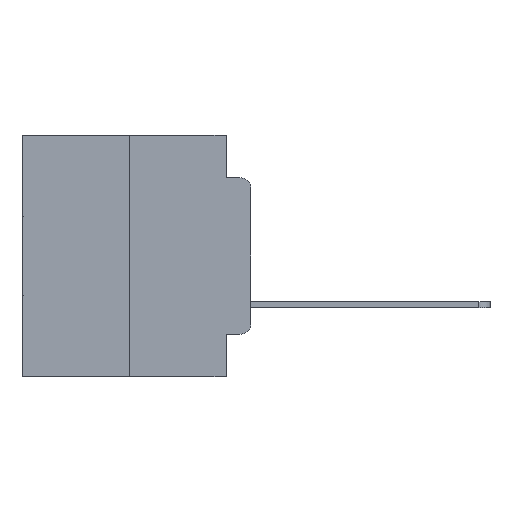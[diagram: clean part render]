
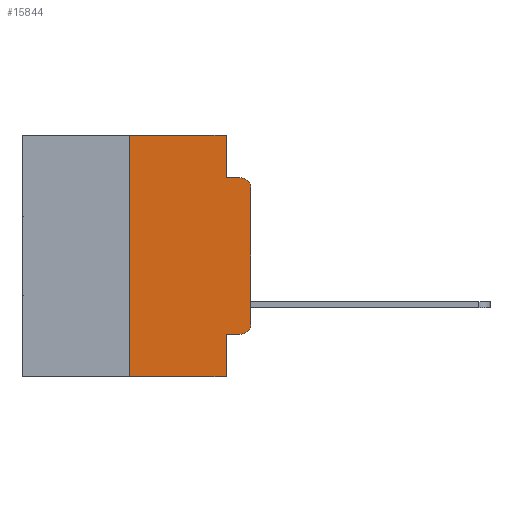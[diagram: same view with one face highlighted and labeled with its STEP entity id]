
A CAD part, left-side view. The second image highlights one B-rep face of the part: STEP entity #15844.
In plain terms, the highlighted planar face has unit normal (-1, 0, 0).
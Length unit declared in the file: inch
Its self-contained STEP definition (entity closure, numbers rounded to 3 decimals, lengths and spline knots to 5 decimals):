
#1087 = LINE ( 'NONE', #21592, #25274 ) ;
#2406 = AXIS2_PLACEMENT_3D ( 'NONE', #21463, #7665, #23724 ) ;
#2684 = CIRCLE ( 'NONE', #2406, 0.02 ) ;
#3044 = VECTOR ( 'NONE', #12171, 39.37008 ) ;
#3562 = EDGE_CURVE ( 'NONE', #9791, #24320, #6657, .T. ) ;
#3823 = LINE ( 'NONE', #4942, #3044 ) ;
#4385 = LINE ( 'NONE', #28917, #22219 ) ;
#4664 = CARTESIAN_POINT ( 'NONE',  ( 0., 0.051, 0. ) ) ;
#4942 = CARTESIAN_POINT ( 'NONE',  ( 0., 0.051, 0. ) ) ;
#5201 = DIRECTION ( 'NONE',  ( 0., 0., 1. ) ) ;
#5294 = EDGE_CURVE ( 'NONE', #24320, #14444, #12164, .T. ) ;
#6011 = EDGE_CURVE ( 'NONE', #27297, #16325, #13536, .T. ) ;
#6657 = CIRCLE ( 'NONE', #10305, 0.02 ) ;
#6861 = VERTEX_POINT ( 'NONE', #24099 ) ;
#6896 = FACE_OUTER_BOUND ( 'NONE', #25706, .T. ) ;
#7262 = VECTOR ( 'NONE', #14156, 39.37008 ) ;
#7665 = DIRECTION ( 'NONE',  ( -1., 0., 0. ) ) ;
#7783 = LINE ( 'NONE', #19919, #13334 ) ;
#7862 = LINE ( 'NONE', #29389, #29689 ) ;
#9021 = ORIENTED_EDGE ( 'NONE', *, *, #5294, .T. ) ;
#9426 = CARTESIAN_POINT ( 'NONE',  ( 0., 0.051, -0.4115 ) ) ;
#9547 = CARTESIAN_POINT ( 'NONE',  ( 0., 0.02, -0.0885 ) ) ;
#9785 = DIRECTION ( 'NONE',  ( 0., 0., -1. ) ) ;
#9791 = VERTEX_POINT ( 'NONE', #19637 ) ;
#9823 = CARTESIAN_POINT ( 'NONE',  ( 0., 0.25, -0.5 ) ) ;
#9932 = CARTESIAN_POINT ( 'NONE',  ( 0., 0., -0.3915 ) ) ;
#10040 = ORIENTED_EDGE ( 'NONE', *, *, #14467, .T. ) ;
#10305 = AXIS2_PLACEMENT_3D ( 'NONE', #21057, #21060, #21267 ) ;
#10607 = PLANE ( 'NONE',  #10878 ) ;
#10878 = AXIS2_PLACEMENT_3D ( 'NONE', #26348, #28483, #15251 ) ;
#11015 = ORIENTED_EDGE ( 'NONE', *, *, #29801, .F. ) ;
#11529 = EDGE_CURVE ( 'NONE', #25397, #9791, #4385, .T. ) ;
#11593 = DIRECTION ( 'NONE',  ( 0., -1., 0. ) ) ;
#12084 = ORIENTED_EDGE ( 'NONE', *, *, #15018, .F. ) ;
#12164 = LINE ( 'NONE', #27948, #16884 ) ;
#12171 = DIRECTION ( 'NONE',  ( 0., 0., -1. ) ) ;
#12251 = CARTESIAN_POINT ( 'NONE',  ( 0., 0., -0.1085 ) ) ;
#12351 = ORIENTED_EDGE ( 'NONE', *, *, #6011, .F. ) ;
#13334 = VECTOR ( 'NONE', #24379, 39.37008 ) ;
#13503 = DIRECTION ( 'NONE',  ( 0., -1., 0. ) ) ;
#13536 = LINE ( 'NONE', #29509, #7262 ) ;
#13708 = VERTEX_POINT ( 'NONE', #18200 ) ;
#13743 = ORIENTED_EDGE ( 'NONE', *, *, #14069, .F. ) ;
#14069 = EDGE_CURVE ( 'NONE', #28813, #27297, #7783, .T. ) ;
#14156 = DIRECTION ( 'NONE',  ( 0., -1., 0. ) ) ;
#14444 = VERTEX_POINT ( 'NONE', #12251 ) ;
#14467 = EDGE_CURVE ( 'NONE', #14444, #20043, #2684, .T. ) ;
#14981 = ORIENTED_EDGE ( 'NONE', *, *, #24403, .T. ) ;
#15018 = EDGE_CURVE ( 'NONE', #16325, #6861, #3823, .T. ) ;
#15251 = DIRECTION ( 'NONE',  ( 0., 0., -1. ) ) ;
#15844 = ADVANCED_FACE ( 'NONE', ( #6896 ), #10607, .F. ) ;
#16325 = VERTEX_POINT ( 'NONE', #4664 ) ;
#16884 = VECTOR ( 'NONE', #5201, 39.37008 ) ;
#17096 = ORIENTED_EDGE ( 'NONE', *, *, #29437, .F. ) ;
#17390 = LINE ( 'NONE', #25580, #28379 ) ;
#17830 = ORIENTED_EDGE ( 'NONE', *, *, #11529, .T. ) ;
#18169 = ORIENTED_EDGE ( 'NONE', *, *, #3562, .T. ) ;
#18200 = CARTESIAN_POINT ( 'NONE',  ( 0., 0.051, -0.5 ) ) ;
#19637 = CARTESIAN_POINT ( 'NONE',  ( 0., 0.02, -0.4115 ) ) ;
#19919 = CARTESIAN_POINT ( 'NONE',  ( 0., 0.25, 0. ) ) ;
#20043 = VERTEX_POINT ( 'NONE', #9547 ) ;
#21057 = CARTESIAN_POINT ( 'NONE',  ( 0., 0.02, -0.3915 ) ) ;
#21060 = DIRECTION ( 'NONE',  ( -1., 0., 0. ) ) ;
#21267 = DIRECTION ( 'NONE',  ( 0., 0., -1. ) ) ;
#21463 = CARTESIAN_POINT ( 'NONE',  ( 0., 0.02, -0.1085 ) ) ;
#21592 = CARTESIAN_POINT ( 'NONE',  ( 0., 0.473, -0.5 ) ) ;
#22115 = DIRECTION ( 'NONE',  ( 0., -1., 0. ) ) ;
#22219 = VECTOR ( 'NONE', #13503, 39.37008 ) ;
#23724 = DIRECTION ( 'NONE',  ( 0., 0., -1. ) ) ;
#24099 = CARTESIAN_POINT ( 'NONE',  ( 0., 0.051, -0.0885 ) ) ;
#24320 = VERTEX_POINT ( 'NONE', #9932 ) ;
#24379 = DIRECTION ( 'NONE',  ( 0., 0., 1. ) ) ;
#24403 = EDGE_CURVE ( 'NONE', #28813, #13708, #1087, .T. ) ;
#25274 = VECTOR ( 'NONE', #22115, 39.37008 ) ;
#25397 = VERTEX_POINT ( 'NONE', #9426 ) ;
#25580 = CARTESIAN_POINT ( 'NONE',  ( 0., 0.051, 0. ) ) ;
#25706 = EDGE_LOOP ( 'NONE', ( #9021, #10040, #11015, #12084, #12351, #13743, #14981, #17096, #17830, #18169 ) ) ;
#26348 = CARTESIAN_POINT ( 'NONE',  ( 0., 0.473, 0. ) ) ;
#27297 = VERTEX_POINT ( 'NONE', #29780 ) ;
#27948 = CARTESIAN_POINT ( 'NONE',  ( 0., 0., 0. ) ) ;
#28379 = VECTOR ( 'NONE', #9785, 39.37008 ) ;
#28483 = DIRECTION ( 'NONE',  ( 1., 0., 0. ) ) ;
#28813 = VERTEX_POINT ( 'NONE', #9823 ) ;
#28917 = CARTESIAN_POINT ( 'NONE',  ( 0., 0.051, -0.4115 ) ) ;
#29389 = CARTESIAN_POINT ( 'NONE',  ( 0., 0.051, -0.0885 ) ) ;
#29437 = EDGE_CURVE ( 'NONE', #25397, #13708, #17390, .T. ) ;
#29509 = CARTESIAN_POINT ( 'NONE',  ( 0., 0.473, 0. ) ) ;
#29689 = VECTOR ( 'NONE', #11593, 39.37008 ) ;
#29780 = CARTESIAN_POINT ( 'NONE',  ( 0., 0.25, 0. ) ) ;
#29801 = EDGE_CURVE ( 'NONE', #6861, #20043, #7862, .T. ) ;
